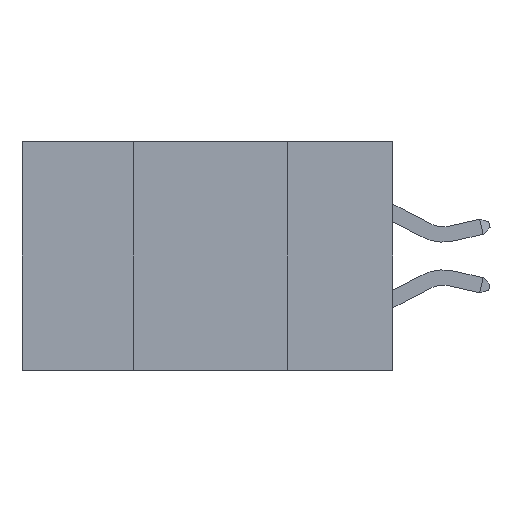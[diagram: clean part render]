
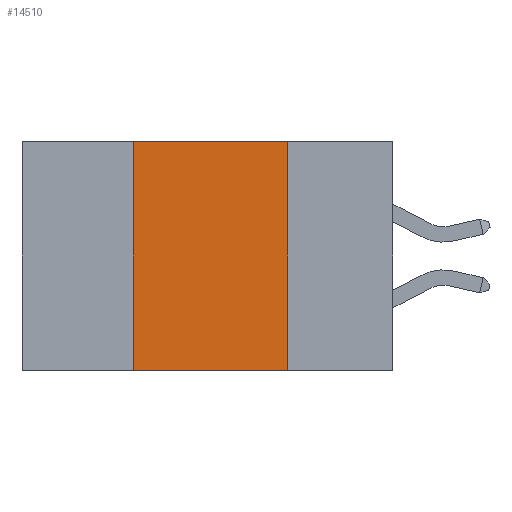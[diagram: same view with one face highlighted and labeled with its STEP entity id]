
A CAD part, left-side view. The second image highlights one B-rep face of the part: STEP entity #14510.
In plain terms, the highlighted planar face has unit normal (-1, 0, 0).
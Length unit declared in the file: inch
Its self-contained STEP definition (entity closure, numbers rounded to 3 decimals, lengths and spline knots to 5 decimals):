
#1087 = EDGE_CURVE ( 'NONE', #7943, #12648, #14691, .T. ) ;
#2720 = LINE ( 'NONE', #25162, #14413 ) ;
#5582 = PLANE ( 'NONE',  #25028 ) ;
#5681 = ORIENTED_EDGE ( 'NONE', *, *, #11258, .F. ) ;
#5972 = CARTESIAN_POINT ( 'NONE',  ( 0., 0.42, -0.37 ) ) ;
#6396 = DIRECTION ( 'NONE',  ( 0., -1., 0. ) ) ;
#6970 = EDGE_CURVE ( 'NONE', #24122, #7757, #14106, .T. ) ;
#7757 = VERTEX_POINT ( 'NONE', #9098 ) ;
#7943 = VERTEX_POINT ( 'NONE', #24019 ) ;
#9098 = CARTESIAN_POINT ( 'NONE',  ( 0., 0.42, 0. ) ) ;
#9660 = CARTESIAN_POINT ( 'NONE',  ( 0., 0.6, 0. ) ) ;
#11044 = ORIENTED_EDGE ( 'NONE', *, *, #22712, .T. ) ;
#11076 = DIRECTION ( 'NONE',  ( 0., 0., -1. ) ) ;
#11258 = EDGE_CURVE ( 'NONE', #7757, #7943, #2720, .T. ) ;
#11884 = DIRECTION ( 'NONE',  ( 0., 0., -1. ) ) ;
#12070 = VECTOR ( 'NONE', #16068, 39.37008 ) ;
#12141 = CARTESIAN_POINT ( 'NONE',  ( 0., 0.6, -0.37 ) ) ;
#12196 = ORIENTED_EDGE ( 'NONE', *, *, #1087, .F. ) ;
#12648 = VERTEX_POINT ( 'NONE', #19183 ) ;
#12683 = LINE ( 'NONE', #12141, #12070 ) ;
#13240 = CARTESIAN_POINT ( 'NONE',  ( 0., 0.17, 0. ) ) ;
#14106 = LINE ( 'NONE', #26439, #23800 ) ;
#14413 = VECTOR ( 'NONE', #6396, 39.37008 ) ;
#14510 = ADVANCED_FACE ( 'NONE', ( #21230 ), #5582, .F. ) ;
#14691 = LINE ( 'NONE', #13240, #25363 ) ;
#16068 = DIRECTION ( 'NONE',  ( 0., -1., 0. ) ) ;
#19183 = CARTESIAN_POINT ( 'NONE',  ( 0., 0.17, -0.37 ) ) ;
#20028 = ORIENTED_EDGE ( 'NONE', *, *, #6970, .F. ) ;
#21230 = FACE_OUTER_BOUND ( 'NONE', #25793, .T. ) ;
#22026 = DIRECTION ( 'NONE',  ( 0., 0., 1. ) ) ;
#22712 = EDGE_CURVE ( 'NONE', #24122, #12648, #12683, .T. ) ;
#23800 = VECTOR ( 'NONE', #22026, 39.37008 ) ;
#24019 = CARTESIAN_POINT ( 'NONE',  ( 0., 0.17, 0. ) ) ;
#24122 = VERTEX_POINT ( 'NONE', #5972 ) ;
#25028 = AXIS2_PLACEMENT_3D ( 'NONE', #9660, #26002, #11884 ) ;
#25162 = CARTESIAN_POINT ( 'NONE',  ( 0., 0.6, 0. ) ) ;
#25363 = VECTOR ( 'NONE', #11076, 39.37008 ) ;
#25793 = EDGE_LOOP ( 'NONE', ( #12196, #5681, #20028, #11044 ) ) ;
#26002 = DIRECTION ( 'NONE',  ( 1., 0., 0. ) ) ;
#26439 = CARTESIAN_POINT ( 'NONE',  ( 0., 0.42, 0. ) ) ;
